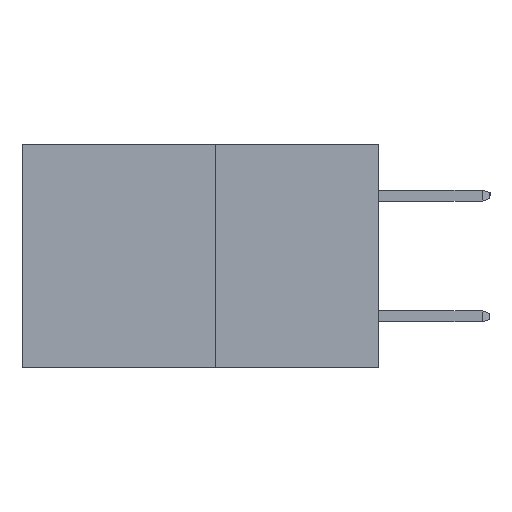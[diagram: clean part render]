
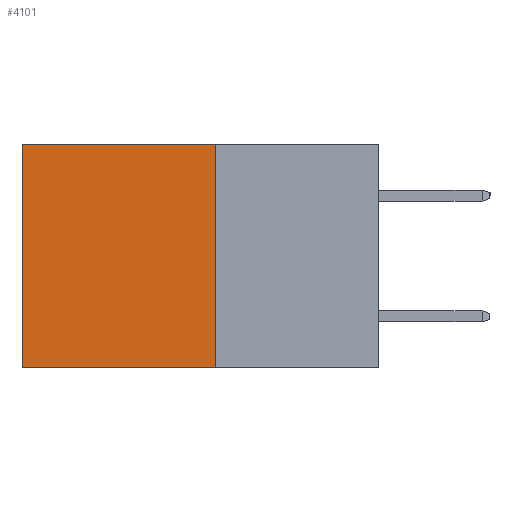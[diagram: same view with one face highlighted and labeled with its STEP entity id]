
A CAD part, left-side view. The second image highlights one B-rep face of the part: STEP entity #4101.
In plain terms, the highlighted planar face has unit normal (-1, 0, 0).
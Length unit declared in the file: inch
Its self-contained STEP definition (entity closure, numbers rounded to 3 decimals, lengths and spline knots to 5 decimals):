
#165 = EDGE_CURVE ( 'NONE', #2433, #7080, #3341, .T. ) ;
#224 = LINE ( 'NONE', #9489, #7916 ) ;
#331 = ORIENTED_EDGE ( 'NONE', *, *, #165, .T. ) ;
#613 = DIRECTION ( 'NONE',  ( 0., 0., -1. ) ) ;
#614 = ORIENTED_EDGE ( 'NONE', *, *, #4168, .F. ) ;
#1018 = VERTEX_POINT ( 'NONE', #7466 ) ;
#1039 = DIRECTION ( 'NONE',  ( 0., 1., 0. ) ) ;
#1253 = VECTOR ( 'NONE', #4752, 39.37008 ) ;
#1373 = LINE ( 'NONE', #4304, #1253 ) ;
#2110 = EDGE_CURVE ( 'NONE', #7080, #1018, #1373, .T. ) ;
#2433 = VERTEX_POINT ( 'NONE', #7324 ) ;
#2724 = EDGE_CURVE ( 'NONE', #7925, #1018, #224, .T. ) ;
#3341 = LINE ( 'NONE', #8586, #5044 ) ;
#4101 = ADVANCED_FACE ( 'NONE', ( #8747 ), #5047, .F. ) ;
#4168 = EDGE_CURVE ( 'NONE', #2433, #7925, #6677, .T. ) ;
#4304 = CARTESIAN_POINT ( 'NONE',  ( 0.277, 0.59, -0.37 ) ) ;
#4338 = DIRECTION ( 'NONE',  ( 0., 0., -1. ) ) ;
#4752 = DIRECTION ( 'NONE',  ( 0., 0., -1. ) ) ;
#4952 = VECTOR ( 'NONE', #613, 39.37008 ) ;
#5044 = VECTOR ( 'NONE', #1039, 39.37008 ) ;
#5047 = PLANE ( 'NONE',  #8115 ) ;
#5182 = DIRECTION ( 'NONE',  ( 0., 1., 0. ) ) ;
#6230 = CARTESIAN_POINT ( 'NONE',  ( 0.277, 0.27, -0.37 ) ) ;
#6627 = CARTESIAN_POINT ( 'NONE',  ( 0.277, 0.27, -0.37 ) ) ;
#6677 = LINE ( 'NONE', #6627, #4952 ) ;
#7066 = CARTESIAN_POINT ( 'NONE',  ( 0.277, 0.27, -0.37 ) ) ;
#7079 = ORIENTED_EDGE ( 'NONE', *, *, #2110, .T. ) ;
#7080 = VERTEX_POINT ( 'NONE', #7991 ) ;
#7324 = CARTESIAN_POINT ( 'NONE',  ( 0.277, 0.27, 0. ) ) ;
#7466 = CARTESIAN_POINT ( 'NONE',  ( 0.277, 0.59, -0.37 ) ) ;
#7916 = VECTOR ( 'NONE', #5182, 39.37008 ) ;
#7925 = VERTEX_POINT ( 'NONE', #6230 ) ;
#7991 = CARTESIAN_POINT ( 'NONE',  ( 0.277, 0.59, 0. ) ) ;
#8115 = AXIS2_PLACEMENT_3D ( 'NONE', #7066, #8651, #4338 ) ;
#8586 = CARTESIAN_POINT ( 'NONE',  ( 0.277, 0.27, 0. ) ) ;
#8651 = DIRECTION ( 'NONE',  ( 1., 0., 0. ) ) ;
#8747 = FACE_OUTER_BOUND ( 'NONE', #8783, .T. ) ;
#8783 = EDGE_LOOP ( 'NONE', ( #7079, #9194, #614, #331 ) ) ;
#9194 = ORIENTED_EDGE ( 'NONE', *, *, #2724, .F. ) ;
#9489 = CARTESIAN_POINT ( 'NONE',  ( 0.277, 0.27, -0.37 ) ) ;
